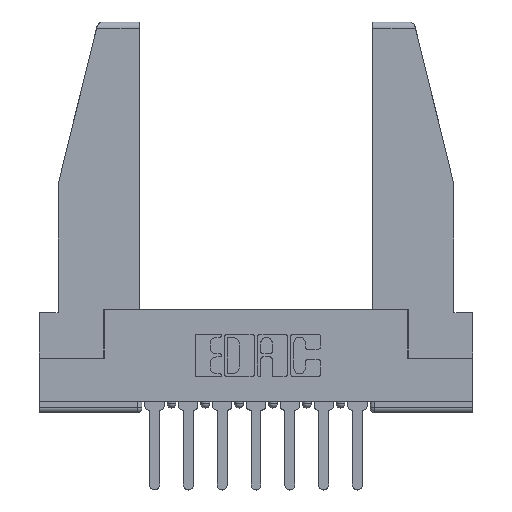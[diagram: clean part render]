
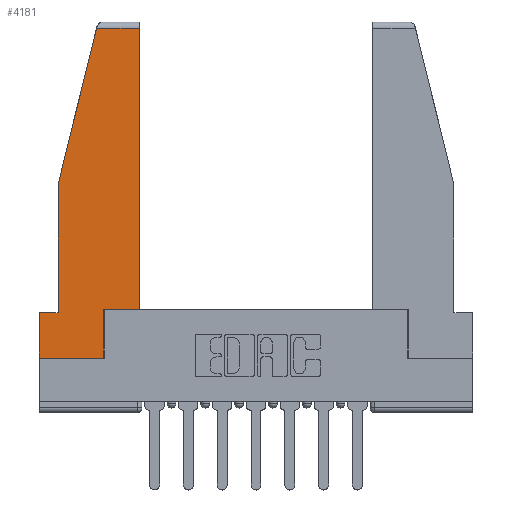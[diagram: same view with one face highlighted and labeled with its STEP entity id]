
A CAD part, top view. The second image highlights one B-rep face of the part: STEP entity #4181.
In plain terms, the highlighted planar face has unit normal (0, 0, 1).
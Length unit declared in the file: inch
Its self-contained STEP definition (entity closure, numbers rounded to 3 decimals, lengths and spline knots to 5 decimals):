
#168 = EDGE_CURVE ( 'NONE', #4767, #3053, #4523, .T. ) ;
#348 = ORIENTED_EDGE ( 'NONE', *, *, #12097, .T. ) ;
#392 = DIRECTION ( 'NONE',  ( 1., 0., 0. ) ) ;
#687 = ORIENTED_EDGE ( 'NONE', *, *, #6724, .T. ) ;
#693 = CARTESIAN_POINT ( 'NONE',  ( 0., 0.21, 0. ) ) ;
#1249 = ORIENTED_EDGE ( 'NONE', *, *, #3854, .T. ) ;
#1372 = CARTESIAN_POINT ( 'NONE',  ( 0., 0., 0. ) ) ;
#1718 = ORIENTED_EDGE ( 'NONE', *, *, #11261, .T. ) ;
#1854 = DIRECTION ( 'NONE',  ( -1., 0., 0. ) ) ;
#2129 = DIRECTION ( 'NONE',  ( -1., 0., 0. ) ) ;
#2238 = ORIENTED_EDGE ( 'NONE', *, *, #8129, .T. ) ;
#2736 = PLANE ( 'NONE',  #10671 ) ;
#2938 = VERTEX_POINT ( 'NONE', #11594 ) ;
#3053 = VERTEX_POINT ( 'NONE', #11792 ) ;
#3132 = VECTOR ( 'NONE', #2129, 39.37008 ) ;
#3184 = VERTEX_POINT ( 'NONE', #11244 ) ;
#3834 = CARTESIAN_POINT ( 'NONE',  ( 0.086, 0.8, 0. ) ) ;
#3854 = EDGE_CURVE ( 'NONE', #10238, #3184, #6837, .T. ) ;
#4181 = ADVANCED_FACE ( 'NONE', ( #4591 ), #2736, .T. ) ;
#4334 = DIRECTION ( 'NONE',  ( 0., 1., 0. ) ) ;
#4347 = VECTOR ( 'NONE', #5484, 39.37008 ) ;
#4399 = LINE ( 'NONE', #11830, #9862 ) ;
#4523 = LINE ( 'NONE', #8438, #8772 ) ;
#4525 = CARTESIAN_POINT ( 'NONE',  ( 0., 0., 0. ) ) ;
#4591 = FACE_OUTER_BOUND ( 'NONE', #7278, .T. ) ;
#4767 = VERTEX_POINT ( 'NONE', #11970 ) ;
#5284 = LINE ( 'NONE', #7137, #10098 ) ;
#5310 = CARTESIAN_POINT ( 'NONE',  ( 0.2636, 1.52, 0. ) ) ;
#5484 = DIRECTION ( 'NONE',  ( 0., 1., 0. ) ) ;
#5541 = EDGE_CURVE ( 'NONE', #10917, #4767, #5548, .T. ) ;
#5548 = LINE ( 'NONE', #11613, #4347 ) ;
#5633 = VECTOR ( 'NONE', #7477, 39.37008 ) ;
#5709 = CARTESIAN_POINT ( 'NONE',  ( 0., 0.21, 0. ) ) ;
#6165 = CARTESIAN_POINT ( 'NONE',  ( 0., 1.52, 0. ) ) ;
#6602 = VECTOR ( 'NONE', #1854, 39.37008 ) ;
#6674 = ORIENTED_EDGE ( 'NONE', *, *, #12166, .T. ) ;
#6724 = EDGE_CURVE ( 'NONE', #12004, #2938, #12304, .T. ) ;
#6837 = LINE ( 'NONE', #3834, #8819 ) ;
#6893 = DIRECTION ( 'NONE',  ( 0., -1., 0. ) ) ;
#7062 = CARTESIAN_POINT ( 'NONE',  ( 0.461, 1.52, 0. ) ) ;
#7083 = ORIENTED_EDGE ( 'NONE', *, *, #168, .T. ) ;
#7137 = CARTESIAN_POINT ( 'NONE',  ( 0.461, 0.223, 0. ) ) ;
#7278 = EDGE_LOOP ( 'NONE', ( #348, #1718, #6674, #1249, #8500, #687, #2238, #10869, #7083 ) ) ;
#7477 = DIRECTION ( 'NONE',  ( 0., -1., 0. ) ) ;
#7599 = VERTEX_POINT ( 'NONE', #5310 ) ;
#7866 = VECTOR ( 'NONE', #392, 39.37008 ) ;
#7940 = CARTESIAN_POINT ( 'NONE',  ( 0.086, 0.8, 0. ) ) ;
#8035 = LINE ( 'NONE', #6165, #3132 ) ;
#8129 = EDGE_CURVE ( 'NONE', #2938, #10917, #10430, .T. ) ;
#8303 = CARTESIAN_POINT ( 'NONE',  ( 0.297, 0., 0. ) ) ;
#8438 = CARTESIAN_POINT ( 'NONE',  ( 0.297, 0.223, 0. ) ) ;
#8439 = DIRECTION ( 'NONE',  ( 0., 0., 1. ) ) ;
#8500 = ORIENTED_EDGE ( 'NONE', *, *, #11520, .T. ) ;
#8772 = VECTOR ( 'NONE', #10748, 39.37008 ) ;
#8819 = VECTOR ( 'NONE', #6893, 39.37008 ) ;
#9605 = CARTESIAN_POINT ( 'NONE',  ( 0., 0.21, 0. ) ) ;
#9862 = VECTOR ( 'NONE', #12196, 39.37008 ) ;
#10098 = VECTOR ( 'NONE', #4334, 39.37008 ) ;
#10238 = VERTEX_POINT ( 'NONE', #7940 ) ;
#10430 = LINE ( 'NONE', #1372, #7866 ) ;
#10671 = AXIS2_PLACEMENT_3D ( 'NONE', #4525, #8439, #12383 ) ;
#10748 = DIRECTION ( 'NONE',  ( 1., 0., 0. ) ) ;
#10869 = ORIENTED_EDGE ( 'NONE', *, *, #5541, .T. ) ;
#10917 = VERTEX_POINT ( 'NONE', #8303 ) ;
#11244 = CARTESIAN_POINT ( 'NONE',  ( 0.086, 0.21, 0. ) ) ;
#11261 = EDGE_CURVE ( 'NONE', #12602, #7599, #8035, .T. ) ;
#11520 = EDGE_CURVE ( 'NONE', #3184, #12004, #12675, .T. ) ;
#11594 = CARTESIAN_POINT ( 'NONE',  ( 0., 0., 0. ) ) ;
#11613 = CARTESIAN_POINT ( 'NONE',  ( 0.297, 0., 0. ) ) ;
#11792 = CARTESIAN_POINT ( 'NONE',  ( 0.461, 0.223, 0. ) ) ;
#11830 = CARTESIAN_POINT ( 'NONE',  ( 0.271, 1.55, 0. ) ) ;
#11970 = CARTESIAN_POINT ( 'NONE',  ( 0.297, 0.223, 0. ) ) ;
#12004 = VERTEX_POINT ( 'NONE', #9605 ) ;
#12097 = EDGE_CURVE ( 'NONE', #3053, #12602, #5284, .T. ) ;
#12166 = EDGE_CURVE ( 'NONE', #7599, #10238, #4399, .T. ) ;
#12196 = DIRECTION ( 'NONE',  ( -0.239, -0.971, 0. ) ) ;
#12304 = LINE ( 'NONE', #693, #5633 ) ;
#12383 = DIRECTION ( 'NONE',  ( 1., 0., 0. ) ) ;
#12602 = VERTEX_POINT ( 'NONE', #7062 ) ;
#12675 = LINE ( 'NONE', #5709, #6602 ) ;
